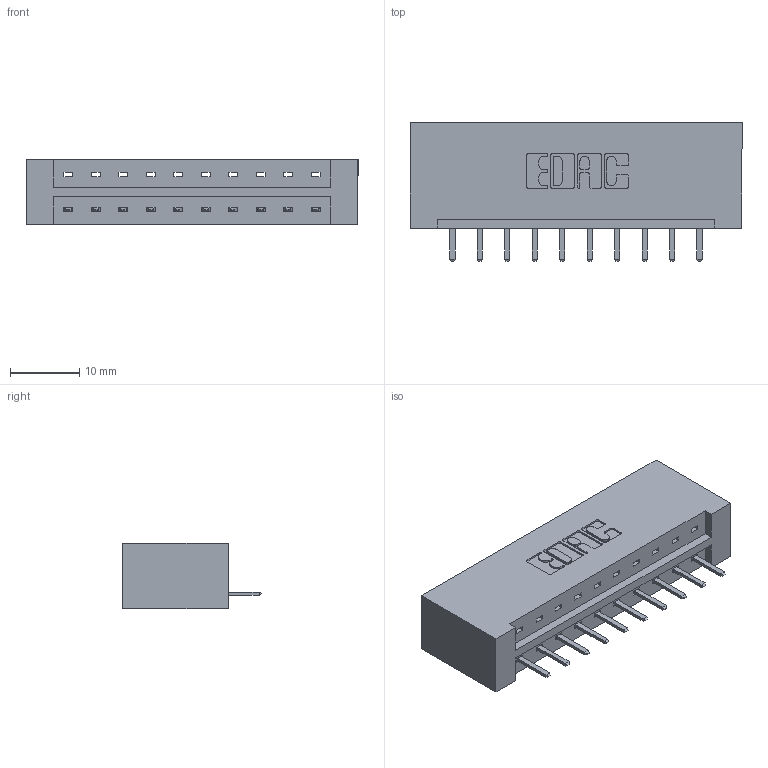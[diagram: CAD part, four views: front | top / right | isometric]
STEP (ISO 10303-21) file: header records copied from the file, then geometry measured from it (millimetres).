
FILE_DESCRIPTION (( 'STEP AP203' ), '1' );
FILE_NAME ('833-010-520-101.STEP', '2020-05-30T18:03:37', ( '' ), ( '' ), 'SwSTEP 2.0', 'SolidWorks 2020', '' );
FILE_SCHEMA (( 'CONFIG_CONTROL_DESIGN' ));
Length unit declared in the file: inch
Products named in the file (3): 833 Part_Lugless; 345-292-001_345-293-120; 833-010-520-101
Assembly tree (11 placements, depth 2):
  833-010-520-101
    833 Part_Lugless
    345-292-001_345-293-120  x10
Bounding box: 47.88 x 20.02 x 9.4 mm (x, y, z)
Volume: 5126.8 mm3; surface area: 5193.2 mm2
Topology: 11 solids, 11 shells, 726 faces, 2127 edges, 1390 vertices
Faces by surface type: plane 506, cylinder 220
Entity records: 10089 total; most frequent: CARTESIAN_POINT 1764, ORIENTED_EDGE 1698, DIRECTION 1533, EDGE_CURVE 849, LINE 725, VECTOR 725, VERTEX_POINT 562, AXIS2_PLACEMENT_3D 404
